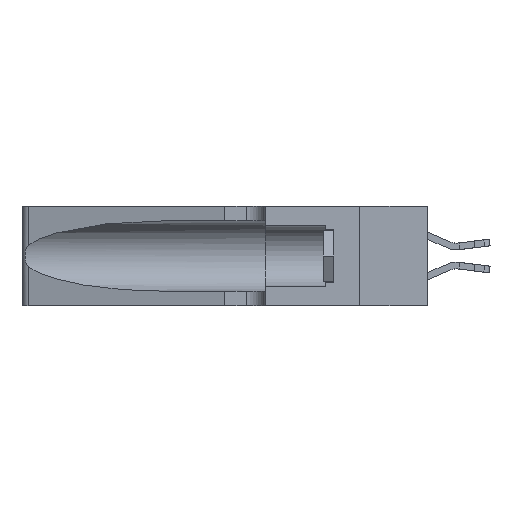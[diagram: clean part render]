
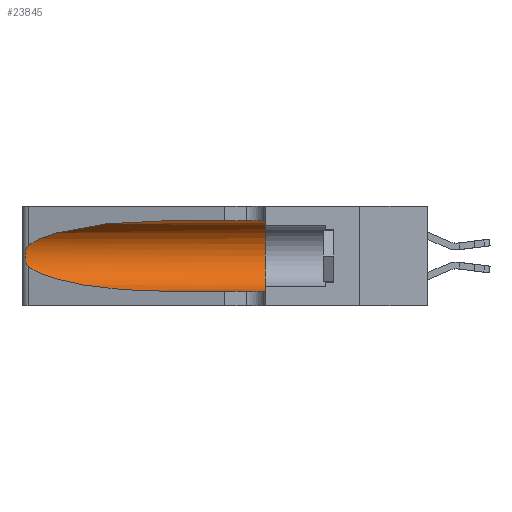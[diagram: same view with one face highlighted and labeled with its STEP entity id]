
A CAD part, left-side view. The second image highlights one B-rep face of the part: STEP entity #23845.
In plain terms, the highlighted cylindrical face has radius 3.308 mm (diameter 6.617 mm), a partial arc.
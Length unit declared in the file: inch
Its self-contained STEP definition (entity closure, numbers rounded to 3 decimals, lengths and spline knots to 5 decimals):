
#389 = CARTESIAN_POINT ( 'NONE',  ( 0.25555, 1.22993, 0.14849 ) ) ;
#595 = CARTESIAN_POINT ( 'NONE',  ( 0.25854, 1.2359, 0.20912 ) ) ;
#1089 = VERTEX_POINT ( 'NONE', #26828 ) ;
#1189 = CARTESIAN_POINT ( 'NONE',  ( 0.18966, 0.96281, 0.05475 ) ) ;
#1451 = FACE_OUTER_BOUND ( 'NONE', #23882, .T. ) ;
#2942 = DIRECTION ( 'NONE',  ( 0., -1., 0. ) ) ;
#3079 = CARTESIAN_POINT ( 'NONE',  ( 0.25487, 1.22718, 0.14631 ) ) ;
#3209 = CARTESIAN_POINT ( 'NONE',  ( 0.18966, 0.96281, 0.31525 ) ) ;
#3268 = EDGE_CURVE ( 'NONE', #1089, #25599, #16372, .T. ) ;
#3339 = LINE ( 'NONE', #26640, #25552 ) ;
#3974 = DIRECTION ( 'NONE',  ( 0., 0., 1. ) ) ;
#5261 = CARTESIAN_POINT ( 'NONE',  ( 0.25639, 1.23184, 0.21858 ) ) ;
#5664 = CARTESIAN_POINT ( 'NONE',  ( 0.25789, 1.23486, 0.15765 ) ) ;
#5900 = ORIENTED_EDGE ( 'NONE', *, *, #16671, .T. ) ;
#6400 = CARTESIAN_POINT ( 'NONE',  ( 0.25487, 1.22718, 0.22369 ) ) ;
#7025 = DIRECTION ( 'NONE',  ( 0., -1., 0. ) ) ;
#7693 = CARTESIAN_POINT ( 'NONE',  ( 0.1305, 0.35, 0.05475 ) ) ;
#8080 = CARTESIAN_POINT ( 'NONE',  ( 0.25487, 1.22718, 0.22369 ) ) ;
#9627 = CYLINDRICAL_SURFACE ( 'NONE', #25004, 0.13025 ) ;
#9757 =( BOUNDED_CURVE ( )  B_SPLINE_CURVE ( 3, ( #25197, #3209, #25301, #8080 ),
 .UNSPECIFIED., .F., .F. ) 
 B_SPLINE_CURVE_WITH_KNOTS ( ( 4, 4 ),
 ( 1.5708, 2.84003 ),
 .UNSPECIFIED. ) 
 CURVE ( )  GEOMETRIC_REPRESENTATION_ITEM ( )  RATIONAL_B_SPLINE_CURVE ( ( 1., 0.87, 0.87, 1. ) ) 
 REPRESENTATION_ITEM ( '' )  );
#10055 = VERTEX_POINT ( 'NONE', #26615 ) ;
#10357 = AXIS2_PLACEMENT_3D ( 'NONE', #13865, #18896, #3974 ) ;
#11059 = CARTESIAN_POINT ( 'NONE',  ( 0.2373, 1.15595, 0.08982 ) ) ;
#11571 = VERTEX_POINT ( 'NONE', #7693 ) ;
#11993 = EDGE_CURVE ( 'NONE', #25599, #11571, #26741, .T. ) ;
#12797 = CARTESIAN_POINT ( 'NONE',  ( 0.1305, 1.61858, 0.31525 ) ) ;
#12942 = CARTESIAN_POINT ( 'NONE',  ( 0.26075, 1.23896, 0.178 ) ) ;
#13047 = CARTESIAN_POINT ( 'NONE',  ( 0.26075, 1.23896, 0.19203 ) ) ;
#13865 = CARTESIAN_POINT ( 'NONE',  ( 0.1305, 0.35, 0.185 ) ) ;
#14010 = CARTESIAN_POINT ( 'NONE',  ( 0.1305, 0.72297, 0.05475 ) ) ;
#14901 = VERTEX_POINT ( 'NONE', #6400 ) ;
#15244 = CARTESIAN_POINT ( 'NONE',  ( 0.25787, 1.23484, 0.2124 ) ) ;
#15309 = ORIENTED_EDGE ( 'NONE', *, *, #17990, .T. ) ;
#15497 =( BOUNDED_CURVE ( )  B_SPLINE_CURVE ( 3, ( #23503, #11059, #1189, #18624 ),
 .UNSPECIFIED., .F., .F. ) 
 B_SPLINE_CURVE_WITH_KNOTS ( ( 4, 4 ),
 ( 3.44316, 4.71239 ),
 .UNSPECIFIED. ) 
 CURVE ( )  GEOMETRIC_REPRESENTATION_ITEM ( )  RATIONAL_B_SPLINE_CURVE ( ( 1., 0.87, 0.87, 1. ) ) 
 REPRESENTATION_ITEM ( '' )  );
#15542 = CARTESIAN_POINT ( 'NONE',  ( 0.25856, 1.23593, 0.16098 ) ) ;
#15569 = VECTOR ( 'NONE', #2942, 39.37008 ) ;
#16022 = DIRECTION ( 'NONE',  ( 0., -1., 0. ) ) ;
#16060 = EDGE_CURVE ( 'NONE', #1089, #14901, #9757, .T. ) ;
#16372 = LINE ( 'NONE', #12797, #15569 ) ;
#16671 = EDGE_CURVE ( 'NONE', #10055, #20176, #15497, .T. ) ;
#17990 = EDGE_CURVE ( 'NONE', #20176, #11571, #3339, .T. ) ;
#18450 = DIRECTION ( 'NONE',  ( 0., 0., -1. ) ) ;
#18624 = CARTESIAN_POINT ( 'NONE',  ( 0.1305, 0.72297, 0.05475 ) ) ;
#18896 = DIRECTION ( 'NONE',  ( 0., 1., 0. ) ) ;
#20176 = VERTEX_POINT ( 'NONE', #14010 ) ;
#20288 = CARTESIAN_POINT ( 'NONE',  ( 0.25555, 1.22994, 0.2215 ) ) ;
#20879 = ORIENTED_EDGE ( 'NONE', *, *, #29105, .T. ) ;
#22184 = ORIENTED_EDGE ( 'NONE', *, *, #16060, .T. ) ;
#23503 = CARTESIAN_POINT ( 'NONE',  ( 0.25487, 1.22718, 0.14631 ) ) ;
#23845 = ADVANCED_FACE ( 'NONE', ( #1451 ), #9627, .F. ) ;
#23882 = EDGE_LOOP ( 'NONE', ( #22184, #20879, #5900, #15309, #28200, #28231 ) ) ;
#25004 = AXIS2_PLACEMENT_3D ( 'NONE', #30706, #16022, #18450 ) ;
#25197 = CARTESIAN_POINT ( 'NONE',  ( 0.1305, 0.72297, 0.31525 ) ) ;
#25301 = CARTESIAN_POINT ( 'NONE',  ( 0.2373, 1.15595, 0.28018 ) ) ;
#25552 = VECTOR ( 'NONE', #7025, 39.37008 ) ;
#25587 = CARTESIAN_POINT ( 'NONE',  ( 0.26017, 1.23833, 0.17102 ) ) ;
#25599 = VERTEX_POINT ( 'NONE', #25872 ) ;
#25872 = CARTESIAN_POINT ( 'NONE',  ( 0.1305, 0.35, 0.31525 ) ) ;
#26615 = CARTESIAN_POINT ( 'NONE',  ( 0.25487, 1.22718, 0.14631 ) ) ;
#26640 = CARTESIAN_POINT ( 'NONE',  ( 0.1305, 1.61858, 0.05475 ) ) ;
#26741 = CIRCLE ( 'NONE', #10357, 0.13025 ) ;
#26828 = CARTESIAN_POINT ( 'NONE',  ( 0.1305, 0.72297, 0.31525 ) ) ;
#27805 = CARTESIAN_POINT ( 'NONE',  ( 0.25639, 1.23186, 0.15144 ) ) ;
#27901 = CARTESIAN_POINT ( 'NONE',  ( 0.26018, 1.23835, 0.19895 ) ) ;
#28200 = ORIENTED_EDGE ( 'NONE', *, *, #11993, .F. ) ;
#28231 = ORIENTED_EDGE ( 'NONE', *, *, #3268, .F. ) ;
#28958 = B_SPLINE_CURVE_WITH_KNOTS ( 'NONE', 3,
 ( #29871, #20288, #5261, #15244, #595, #27901, #13047, #12942, #25587, #15542, #5664, #27805, #389, #3079 ),
 .UNSPECIFIED., .F., .F.,
 ( 4, 2, 2, 2, 2, 2, 4 ),
 ( 0., 0.00027, 0.00053, 0.00107, 0.0016, 0.00187, 0.00214 ),
 .UNSPECIFIED. ) ;
#29105 = EDGE_CURVE ( 'NONE', #14901, #10055, #28958, .T. ) ;
#29871 = CARTESIAN_POINT ( 'NONE',  ( 0.25487, 1.22718, 0.22369 ) ) ;
#30706 = CARTESIAN_POINT ( 'NONE',  ( 0.1305, 1.61858, 0.185 ) ) ;
